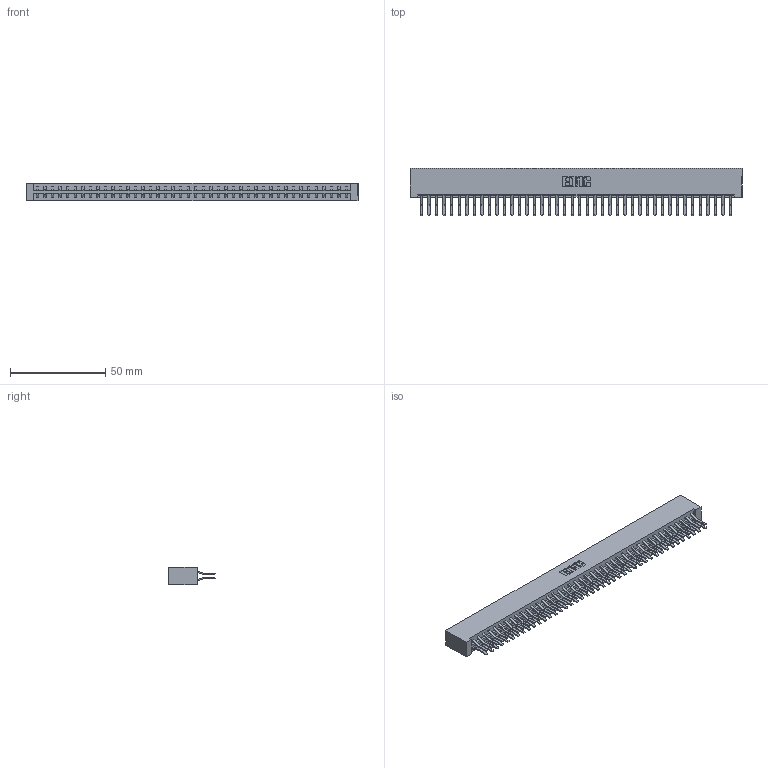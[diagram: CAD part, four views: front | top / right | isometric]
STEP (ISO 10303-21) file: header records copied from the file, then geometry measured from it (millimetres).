
FILE_DESCRIPTION (( 'STEP AP203' ), '1' );
FILE_NAME ('833-084-560-201.STEP', '2020-06-06T02:26:46', ( '' ), ( '' ), 'SwSTEP 2.0', 'SolidWorks 2020', '' );
FILE_SCHEMA (( 'CONFIG_CONTROL_DESIGN' ));
Length unit declared in the file: inch
Products named in the file (3): 345-292-001_560 Tail; 833 Part_Lugless; 833-084-560-201
Assembly tree (85 placements, depth 2):
  833-084-560-201
    833 Part_Lugless
    345-292-001_560 Tail  x84
Bounding box: 174.68 x 24.78 x 9.4 mm (x, y, z)
Volume: 19016.2 mm3; surface area: 24076.9 mm2
Topology: 85 solids, 85 shells, 4642 faces, 13811 edges, 9094 vertices
Faces by surface type: plane 3090, cylinder 1552
Entity records: 26831 total; most frequent: CARTESIAN_POINT 4446, ORIENTED_EDGE 4382, DIRECTION 3795, EDGE_CURVE 2191, LINE 2067, VECTOR 2067, VERTEX_POINT 1458, AXIS2_PLACEMENT_3D 864
